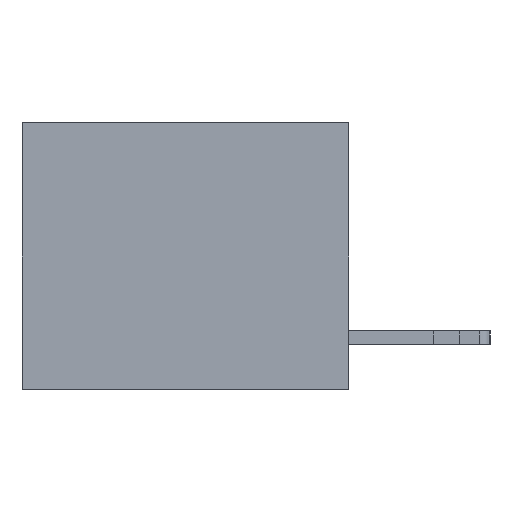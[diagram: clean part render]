
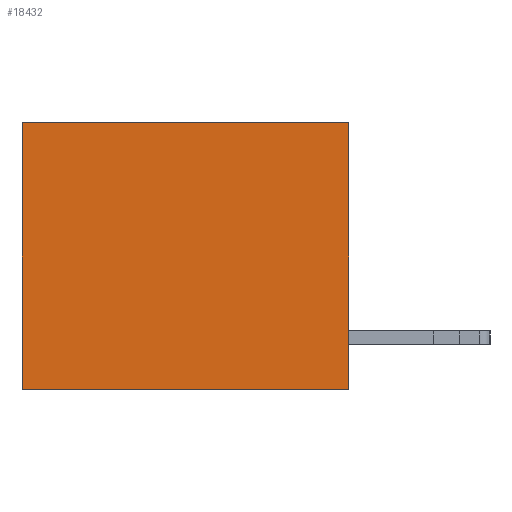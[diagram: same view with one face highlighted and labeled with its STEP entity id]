
A CAD part, left-side view. The second image highlights one B-rep face of the part: STEP entity #18432.
In plain terms, the highlighted planar face has unit normal (-1, 0, 0).
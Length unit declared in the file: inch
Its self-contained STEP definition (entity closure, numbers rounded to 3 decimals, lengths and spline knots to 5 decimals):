
#455 = VERTEX_POINT ( 'NONE', #20240 ) ;
#532 = EDGE_CURVE ( 'NONE', #7086, #455, #22888, .T. ) ;
#1059 = ORIENTED_EDGE ( 'NONE', *, *, #11498, .T. ) ;
#1080 = DIRECTION ( 'NONE',  ( 0., 1., 0. ) ) ;
#1934 = EDGE_CURVE ( 'NONE', #4859, #4842, #6272, .T. ) ;
#2181 = VECTOR ( 'NONE', #6234, 39.37008 ) ;
#2832 = EDGE_CURVE ( 'NONE', #455, #4842, #13902, .T. ) ;
#3777 = LINE ( 'NONE', #10926, #19365 ) ;
#4842 = VERTEX_POINT ( 'NONE', #19230 ) ;
#4859 = VERTEX_POINT ( 'NONE', #21453 ) ;
#6234 = DIRECTION ( 'NONE',  ( 0., 0., -1. ) ) ;
#6272 = LINE ( 'NONE', #24657, #2181 ) ;
#6451 = ORIENTED_EDGE ( 'NONE', *, *, #532, .F. ) ;
#7086 = VERTEX_POINT ( 'NONE', #9101 ) ;
#7629 = VECTOR ( 'NONE', #24427, 39.37008 ) ;
#8220 = CARTESIAN_POINT ( 'NONE',  ( 0.3165, 0., -0.49 ) ) ;
#8334 = ORIENTED_EDGE ( 'NONE', *, *, #2832, .F. ) ;
#8460 = VECTOR ( 'NONE', #14848, 39.37008 ) ;
#9101 = CARTESIAN_POINT ( 'NONE',  ( 0.3165, 0., 0. ) ) ;
#10872 = FACE_OUTER_BOUND ( 'NONE', #20354, .T. ) ;
#10926 = CARTESIAN_POINT ( 'NONE',  ( 0.3165, 0., 0. ) ) ;
#11498 = EDGE_CURVE ( 'NONE', #7086, #4859, #3777, .T. ) ;
#13902 = LINE ( 'NONE', #22900, #8460 ) ;
#14118 = CARTESIAN_POINT ( 'NONE',  ( 0.3165, 0., -0.49 ) ) ;
#14367 = PLANE ( 'NONE',  #24515 ) ;
#14848 = DIRECTION ( 'NONE',  ( 0., 1., 0. ) ) ;
#18432 = ADVANCED_FACE ( 'NONE', ( #10872 ), #14367, .F. ) ;
#19230 = CARTESIAN_POINT ( 'NONE',  ( 0.3165, 0.6, -0.49 ) ) ;
#19365 = VECTOR ( 'NONE', #1080, 39.37008 ) ;
#20240 = CARTESIAN_POINT ( 'NONE',  ( 0.3165, 0., -0.49 ) ) ;
#20354 = EDGE_LOOP ( 'NONE', ( #22332, #8334, #6451, #1059 ) ) ;
#21453 = CARTESIAN_POINT ( 'NONE',  ( 0.3165, 0.6, 0. ) ) ;
#22332 = ORIENTED_EDGE ( 'NONE', *, *, #1934, .T. ) ;
#22888 = LINE ( 'NONE', #8220, #7629 ) ;
#22900 = CARTESIAN_POINT ( 'NONE',  ( 0.3165, 0., -0.49 ) ) ;
#23143 = DIRECTION ( 'NONE',  ( 0., 0., -1. ) ) ;
#24427 = DIRECTION ( 'NONE',  ( 0., 0., -1. ) ) ;
#24515 = AXIS2_PLACEMENT_3D ( 'NONE', #14118, #25012, #23143 ) ;
#24657 = CARTESIAN_POINT ( 'NONE',  ( 0.3165, 0.6, -0.49 ) ) ;
#25012 = DIRECTION ( 'NONE',  ( 1., 0., 0. ) ) ;
